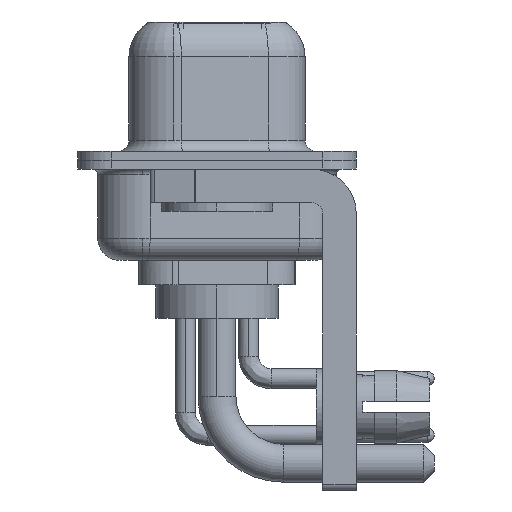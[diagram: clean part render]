
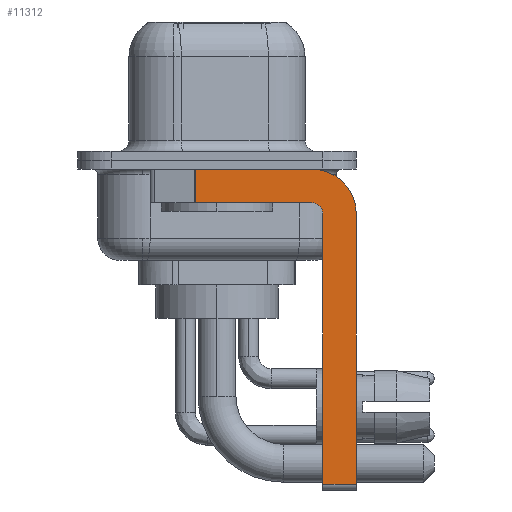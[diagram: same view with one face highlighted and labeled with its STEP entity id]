
A CAD part, left-side view. The second image highlights one B-rep face of the part: STEP entity #11312.
In plain terms, the highlighted planar face has unit normal (-1, 0, 0).
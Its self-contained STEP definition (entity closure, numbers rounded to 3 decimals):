
#153 = VECTOR ( 'NONE', #17063, 1000. ) ;
#162 = CARTESIAN_POINT ( 'NONE',  ( -2.9, -4.25, -0.4 ) ) ;
#652 = VECTOR ( 'NONE', #5891, 1000. ) ;
#754 = CARTESIAN_POINT ( 'NONE',  ( -2.9, -4.25, -14.55 ) ) ;
#1035 = DIRECTION ( 'NONE',  ( 0., 0., 1. ) ) ;
#1468 = ORIENTED_EDGE ( 'NONE', *, *, #17756, .T. ) ;
#1552 = DIRECTION ( 'NONE',  ( 0., 0., -1. ) ) ;
#1706 = DIRECTION ( 'NONE',  ( 0., 1., 0. ) ) ;
#1971 = EDGE_CURVE ( 'NONE', #25381, #16227, #16067, .T. ) ;
#2442 = VERTEX_POINT ( 'NONE', #19277 ) ;
#2509 = VERTEX_POINT ( 'NONE', #13814 ) ;
#3521 = DIRECTION ( 'NONE',  ( 1., 0., 0. ) ) ;
#3561 = CARTESIAN_POINT ( 'NONE',  ( -2.9, -4.25, -1.9 ) ) ;
#3652 = FACE_OUTER_BOUND ( 'NONE', #16310, .T. ) ;
#3769 = DIRECTION ( 'NONE',  ( 0., 0., -1. ) ) ;
#4032 = CARTESIAN_POINT ( 'NONE',  ( -2.9, -6.25, -2.4 ) ) ;
#4629 = LINE ( 'NONE', #23303, #16721 ) ;
#4990 = DIRECTION ( 'NONE',  ( -1., 0., 0. ) ) ;
#5387 = EDGE_CURVE ( 'NONE', #15786, #10595, #12273, .T. ) ;
#5891 = DIRECTION ( 'NONE',  ( 0., 0., -1. ) ) ;
#5953 = ORIENTED_EDGE ( 'NONE', *, *, #5387, .F. ) ;
#6475 = CARTESIAN_POINT ( 'NONE',  ( -2.9, 3., -0.4 ) ) ;
#6748 = AXIS2_PLACEMENT_3D ( 'NONE', #9362, #4990, #17456 ) ;
#7616 = EDGE_CURVE ( 'NONE', #2442, #19073, #24633, .T. ) ;
#7782 = EDGE_CURVE ( 'NONE', #2509, #25381, #4629, .T. ) ;
#7922 = EDGE_CURVE ( 'NONE', #19073, #15786, #11069, .T. ) ;
#8070 = DIRECTION ( 'NONE',  ( 0., -1., 0. ) ) ;
#9362 = CARTESIAN_POINT ( 'NONE',  ( -2.9, -4.25, -2.4 ) ) ;
#9410 = LINE ( 'NONE', #3561, #11463 ) ;
#10595 = VERTEX_POINT ( 'NONE', #12346 ) ;
#11069 = CIRCLE ( 'NONE', #20803, 2. ) ;
#11111 = VECTOR ( 'NONE', #8070, 1000. ) ;
#11312 = ADVANCED_FACE ( 'NONE', ( #3652 ), #12022, .F. ) ;
#11463 = VECTOR ( 'NONE', #1706, 1000. ) ;
#11644 = CARTESIAN_POINT ( 'NONE',  ( -2.9, -4.25, -2.4 ) ) ;
#11756 = CARTESIAN_POINT ( 'NONE',  ( -2.9, -4.25, -2.4 ) ) ;
#12022 = PLANE ( 'NONE',  #16826 ) ;
#12064 = CARTESIAN_POINT ( 'NONE',  ( -2.9, -6.25, -2.4 ) ) ;
#12273 = LINE ( 'NONE', #4032, #652 ) ;
#12274 = ORIENTED_EDGE ( 'NONE', *, *, #18385, .T. ) ;
#12346 = CARTESIAN_POINT ( 'NONE',  ( -2.9, -6.25, -14.55 ) ) ;
#13611 = DIRECTION ( 'NONE',  ( 1., 0., 0. ) ) ;
#13709 = LINE ( 'NONE', #17578, #24251 ) ;
#13814 = CARTESIAN_POINT ( 'NONE',  ( -2.9, -4.75, -14.55 ) ) ;
#14088 = EDGE_CURVE ( 'NONE', #16227, #14383, #9410, .T. ) ;
#14383 = VERTEX_POINT ( 'NONE', #24492 ) ;
#14652 = ORIENTED_EDGE ( 'NONE', *, *, #7782, .F. ) ;
#14922 = CARTESIAN_POINT ( 'NONE',  ( -2.9, -4.25, -1.9 ) ) ;
#15786 = VERTEX_POINT ( 'NONE', #12064 ) ;
#16067 = CIRCLE ( 'NONE', #6748, 0.5 ) ;
#16227 = VERTEX_POINT ( 'NONE', #14922 ) ;
#16310 = EDGE_LOOP ( 'NONE', ( #24900, #1468, #21855, #17395, #14652, #12274, #5953, #17888 ) ) ;
#16721 = VECTOR ( 'NONE', #1035, 1000. ) ;
#16826 = AXIS2_PLACEMENT_3D ( 'NONE', #11756, #3521, #26048 ) ;
#17063 = DIRECTION ( 'NONE',  ( 0., -1., 0. ) ) ;
#17375 = CARTESIAN_POINT ( 'NONE',  ( -2.9, -4.75, -2.4 ) ) ;
#17395 = ORIENTED_EDGE ( 'NONE', *, *, #1971, .F. ) ;
#17456 = DIRECTION ( 'NONE',  ( 0., 0., 1. ) ) ;
#17578 = CARTESIAN_POINT ( 'NONE',  ( -2.9, 0.978, -1.9 ) ) ;
#17756 = EDGE_CURVE ( 'NONE', #2442, #14383, #13709, .T. ) ;
#17888 = ORIENTED_EDGE ( 'NONE', *, *, #7922, .F. ) ;
#18385 = EDGE_CURVE ( 'NONE', #2509, #10595, #19178, .T. ) ;
#19073 = VERTEX_POINT ( 'NONE', #162 ) ;
#19178 = LINE ( 'NONE', #754, #153 ) ;
#19277 = CARTESIAN_POINT ( 'NONE',  ( -2.9, 0.978, -0.4 ) ) ;
#20803 = AXIS2_PLACEMENT_3D ( 'NONE', #11644, #13611, #1552 ) ;
#21855 = ORIENTED_EDGE ( 'NONE', *, *, #14088, .F. ) ;
#23303 = CARTESIAN_POINT ( 'NONE',  ( -2.9, -4.75, -14.8 ) ) ;
#24251 = VECTOR ( 'NONE', #3769, 1000. ) ;
#24492 = CARTESIAN_POINT ( 'NONE',  ( -2.9, 0.978, -1.9 ) ) ;
#24633 = LINE ( 'NONE', #6475, #11111 ) ;
#24900 = ORIENTED_EDGE ( 'NONE', *, *, #7616, .F. ) ;
#25381 = VERTEX_POINT ( 'NONE', #17375 ) ;
#26048 = DIRECTION ( 'NONE',  ( 0., 0., -1. ) ) ;
